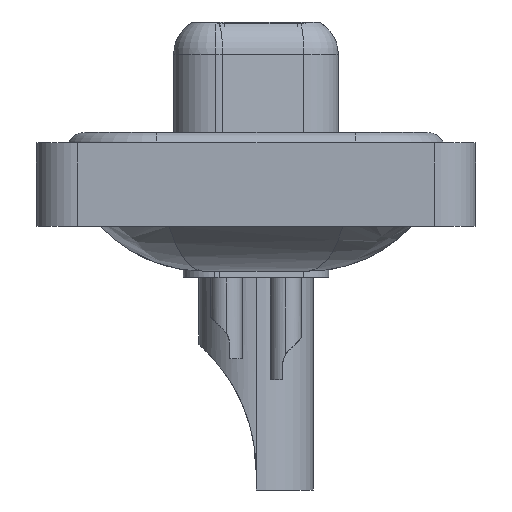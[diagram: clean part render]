
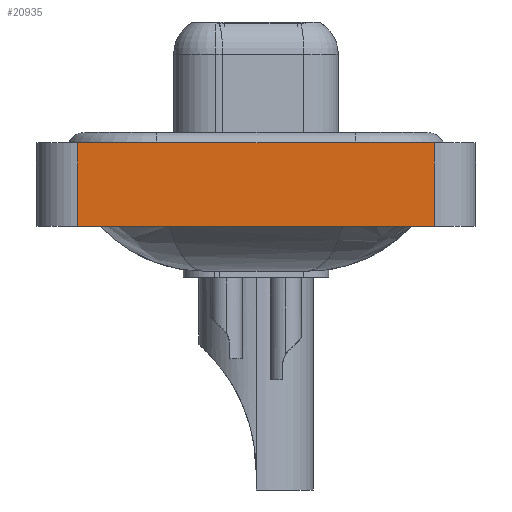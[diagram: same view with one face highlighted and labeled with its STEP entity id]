
A CAD part, left-side view. The second image highlights one B-rep face of the part: STEP entity #20935.
In plain terms, the highlighted planar face has unit normal (-1, 0, 0).
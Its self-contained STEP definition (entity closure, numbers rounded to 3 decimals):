
#433 = LINE ( 'NONE', #10938, #22710 ) ;
#696 = CARTESIAN_POINT ( 'NONE',  ( -7.35, 8.55, 0.4 ) ) ;
#1348 = CARTESIAN_POINT ( 'NONE',  ( -7.35, -8.55, -3.6 ) ) ;
#1678 = VECTOR ( 'NONE', #25021, 1000. ) ;
#2266 = ORIENTED_EDGE ( 'NONE', *, *, #9723, .T. ) ;
#2454 = ORIENTED_EDGE ( 'NONE', *, *, #14005, .F. ) ;
#3112 = PLANE ( 'NONE',  #17593 ) ;
#3365 = DIRECTION ( 'NONE',  ( 0., -1., 0. ) ) ;
#4647 = VERTEX_POINT ( 'NONE', #26531 ) ;
#7444 = DIRECTION ( 'NONE',  ( 0., 0., 1. ) ) ;
#9317 = CARTESIAN_POINT ( 'NONE',  ( -7.35, -8.55, -3.6 ) ) ;
#9659 = VECTOR ( 'NONE', #3365, 1000. ) ;
#9723 = EDGE_CURVE ( 'NONE', #25648, #4647, #25439, .T. ) ;
#10938 = CARTESIAN_POINT ( 'NONE',  ( -7.35, 8.55, -3.6 ) ) ;
#12807 = DIRECTION ( 'NONE',  ( 0., 0., 1. ) ) ;
#12842 = LINE ( 'NONE', #24751, #1678 ) ;
#13333 = EDGE_CURVE ( 'NONE', #25313, #25648, #24513, .T. ) ;
#14005 = EDGE_CURVE ( 'NONE', #26287, #4647, #12842, .T. ) ;
#15524 = VECTOR ( 'NONE', #25569, 1000. ) ;
#16633 = ORIENTED_EDGE ( 'NONE', *, *, #20759, .F. ) ;
#17593 = AXIS2_PLACEMENT_3D ( 'NONE', #9317, #20081, #7444 ) ;
#19662 = CARTESIAN_POINT ( 'NONE',  ( -7.35, -8.55, -3.6 ) ) ;
#20081 = DIRECTION ( 'NONE',  ( -1., 0., 0. ) ) ;
#20611 = EDGE_LOOP ( 'NONE', ( #2266, #2454, #16633, #24208 ) ) ;
#20759 = EDGE_CURVE ( 'NONE', #25313, #26287, #433, .T. ) ;
#20881 = CARTESIAN_POINT ( 'NONE',  ( -7.35, 8.55, -3.6 ) ) ;
#20935 = ADVANCED_FACE ( 'NONE', ( #25927 ), #3112, .T. ) ;
#22710 = VECTOR ( 'NONE', #12807, 1000. ) ;
#24208 = ORIENTED_EDGE ( 'NONE', *, *, #13333, .T. ) ;
#24513 = LINE ( 'NONE', #1348, #9659 ) ;
#24751 = CARTESIAN_POINT ( 'NONE',  ( -7.35, -8.55, 0.4 ) ) ;
#25021 = DIRECTION ( 'NONE',  ( 0., -1., 0. ) ) ;
#25313 = VERTEX_POINT ( 'NONE', #20881 ) ;
#25439 = LINE ( 'NONE', #25834, #15524 ) ;
#25569 = DIRECTION ( 'NONE',  ( 0., 0., 1. ) ) ;
#25648 = VERTEX_POINT ( 'NONE', #19662 ) ;
#25834 = CARTESIAN_POINT ( 'NONE',  ( -7.35, -8.55, -3.6 ) ) ;
#25927 = FACE_OUTER_BOUND ( 'NONE', #20611, .T. ) ;
#26287 = VERTEX_POINT ( 'NONE', #696 ) ;
#26531 = CARTESIAN_POINT ( 'NONE',  ( -7.35, -8.55, 0.4 ) ) ;
